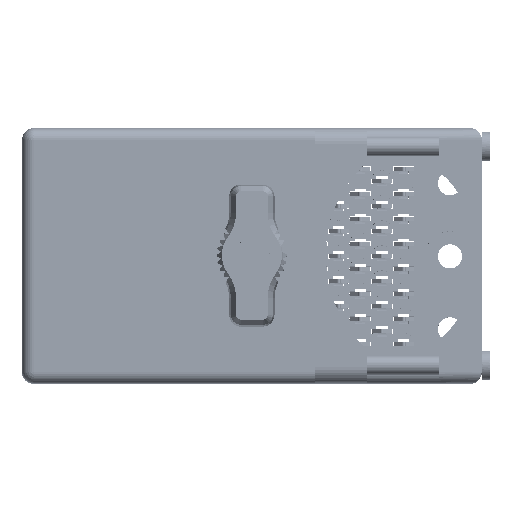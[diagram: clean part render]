
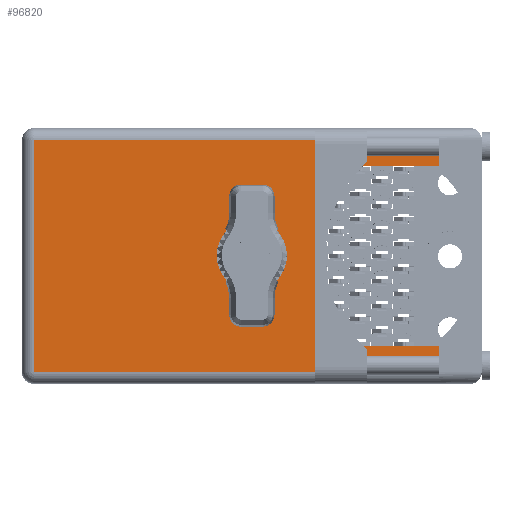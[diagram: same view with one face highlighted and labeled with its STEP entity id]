
A CAD part, top view. The second image highlights one B-rep face of the part: STEP entity #96820.
In plain terms, the highlighted face is planar.
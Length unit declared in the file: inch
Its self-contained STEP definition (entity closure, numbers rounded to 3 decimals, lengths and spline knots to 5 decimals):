
#288 = EDGE_CURVE ( 'NONE', #86348, #95004, #94879, .T. ) ;
#524 = CARTESIAN_POINT ( 'NONE',  ( 1.1215, 1.93, 0.54 ) ) ;
#705 = CARTESIAN_POINT ( 'NONE',  ( 1.1215, 1.93, 0.695 ) ) ;
#796 = ORIENTED_EDGE ( 'NONE', *, *, #88542, .T. ) ;
#2983 = VERTEX_POINT ( 'NONE', #27472 ) ;
#4107 = DIRECTION ( 'NONE',  ( -1., 0., 0. ) ) ;
#4232 = VECTOR ( 'NONE', #84432, 39.37008 ) ;
#4246 = CARTESIAN_POINT ( 'NONE',  ( 1.1215, 1.93, 0.54 ) ) ;
#7202 = DIRECTION ( 'NONE',  ( 1., 0., 0. ) ) ;
#8915 = CARTESIAN_POINT ( 'NONE',  ( 1.1215, 1.93, 0.695 ) ) ;
#9137 = DIRECTION ( 'NONE',  ( 0., 1., 0. ) ) ;
#14262 = VERTEX_POINT ( 'NONE', #8915 ) ;
#14741 = CARTESIAN_POINT ( 'NONE',  ( 0.4075, 1.93, 0.54 ) ) ;
#14955 = CARTESIAN_POINT ( 'NONE',  ( 0., 1.93, 0. ) ) ;
#16380 = ORIENTED_EDGE ( 'NONE', *, *, #67704, .T. ) ;
#16531 = ORIENTED_EDGE ( 'NONE', *, *, #102287, .T. ) ;
#17301 = DIRECTION ( 'NONE',  ( 0., 0., 1. ) ) ;
#17401 = EDGE_CURVE ( 'NONE', #102230, #2983, #83563, .T. ) ;
#18575 = CARTESIAN_POINT ( 'NONE',  ( 1.1215, 1.93, -0.765 ) ) ;
#19406 = VECTOR ( 'NONE', #26752, 39.37008 ) ;
#21004 = EDGE_LOOP ( 'NONE', ( #67143, #16531, #27596, #26174, #79886, #796, #93808, #16380 ) ) ;
#21429 = AXIS2_PLACEMENT_3D ( 'NONE', #82917, #9137, #17301 ) ;
#23336 = CARTESIAN_POINT ( 'NONE',  ( -1.3075, 1.93, -0.695 ) ) ;
#24018 = CARTESIAN_POINT ( 'NONE',  ( 0.4075, 1.93, -0.54 ) ) ;
#24276 = LINE ( 'NONE', #4246, #86844 ) ;
#25543 = ORIENTED_EDGE ( 'NONE', *, *, #105712, .F. ) ;
#25578 = DIRECTION ( 'NONE',  ( 0., 1., 0. ) ) ;
#26174 = ORIENTED_EDGE ( 'NONE', *, *, #61671, .T. ) ;
#26287 = DIRECTION ( 'NONE',  ( 0., 0., -1. ) ) ;
#26752 = DIRECTION ( 'NONE',  ( 1., 0., 0. ) ) ;
#27472 = CARTESIAN_POINT ( 'NONE',  ( 1.1215, 1.93, -0.54 ) ) ;
#27596 = ORIENTED_EDGE ( 'NONE', *, *, #50671, .F. ) ;
#31166 = DIRECTION ( 'NONE',  ( 0., 0., 1. ) ) ;
#34986 = DIRECTION ( 'NONE',  ( 0., 0., 1. ) ) ;
#36555 = PLANE ( 'NONE',  #62351 ) ;
#38083 = CARTESIAN_POINT ( 'NONE',  ( 0., 1.93, -0.17 ) ) ;
#39575 = LINE ( 'NONE', #705, #86782 ) ;
#39820 = EDGE_CURVE ( 'NONE', #99086, #43761, #62608, .T. ) ;
#40971 = CARTESIAN_POINT ( 'NONE',  ( 0., 1.93, 0.17 ) ) ;
#43761 = VERTEX_POINT ( 'NONE', #40971 ) ;
#48873 = VERTEX_POINT ( 'NONE', #524 ) ;
#49514 = LINE ( 'NONE', #69487, #53287 ) ;
#49958 = LINE ( 'NONE', #91996, #19406 ) ;
#50575 = ORIENTED_EDGE ( 'NONE', *, *, #39820, .F. ) ;
#50671 = EDGE_CURVE ( 'NONE', #48873, #14262, #61589, .T. ) ;
#52923 = DIRECTION ( 'NONE',  ( 0., 1., 0. ) ) ;
#53287 = VECTOR ( 'NONE', #85225, 39.37008 ) ;
#60062 = DIRECTION ( 'NONE',  ( 0., 0., 1. ) ) ;
#61589 = LINE ( 'NONE', #92238, #4232 ) ;
#61671 = EDGE_CURVE ( 'NONE', #48873, #86348, #24276, .T. ) ;
#62351 = AXIS2_PLACEMENT_3D ( 'NONE', #101777, #52923, #4107 ) ;
#62608 = CIRCLE ( 'NONE', #21429, 0.17 ) ;
#64220 = EDGE_LOOP ( 'NONE', ( #25543, #50575 ) ) ;
#65698 = CIRCLE ( 'NONE', #90373, 0.17 ) ;
#67143 = ORIENTED_EDGE ( 'NONE', *, *, #95298, .T. ) ;
#67704 = EDGE_CURVE ( 'NONE', #102230, #101703, #49514, .T. ) ;
#68015 = DIRECTION ( 'NONE',  ( -1., 0., 0. ) ) ;
#69487 = CARTESIAN_POINT ( 'NONE',  ( -1.3775, 1.93, -0.695 ) ) ;
#72274 = FACE_BOUND ( 'NONE', #64220, .T. ) ;
#73155 = VECTOR ( 'NONE', #26287, 39.37008 ) ;
#74495 = VECTOR ( 'NONE', #34986, 39.37008 ) ;
#74748 = FACE_OUTER_BOUND ( 'NONE', #21004, .T. ) ;
#79886 = ORIENTED_EDGE ( 'NONE', *, *, #288, .T. ) ;
#80039 = CARTESIAN_POINT ( 'NONE',  ( -1.3075, 1.93, -0.765 ) ) ;
#80666 = CARTESIAN_POINT ( 'NONE',  ( 1.1215, 1.93, -0.695 ) ) ;
#82917 = CARTESIAN_POINT ( 'NONE',  ( 0., 1.93, 0. ) ) ;
#83563 = LINE ( 'NONE', #18575, #74495 ) ;
#84432 = DIRECTION ( 'NONE',  ( 0., 0., 1. ) ) ;
#85225 = DIRECTION ( 'NONE',  ( -1., 0., 0. ) ) ;
#86348 = VERTEX_POINT ( 'NONE', #14741 ) ;
#86782 = VECTOR ( 'NONE', #7202, 39.37008 ) ;
#86844 = VECTOR ( 'NONE', #68015, 39.37008 ) ;
#88542 = EDGE_CURVE ( 'NONE', #95004, #2983, #49958, .T. ) ;
#90373 = AXIS2_PLACEMENT_3D ( 'NONE', #14955, #25578, #60062 ) ;
#90452 = VECTOR ( 'NONE', #31166, 39.37008 ) ;
#91663 = LINE ( 'NONE', #80039, #90452 ) ;
#91996 = CARTESIAN_POINT ( 'NONE',  ( 1.1215, 1.93, -0.54 ) ) ;
#92238 = CARTESIAN_POINT ( 'NONE',  ( 1.1215, 1.93, -0.765 ) ) ;
#92940 = CARTESIAN_POINT ( 'NONE',  ( 0.4075, 1.93, -0.54 ) ) ;
#93277 = CARTESIAN_POINT ( 'NONE',  ( -1.3075, 1.93, 0.695 ) ) ;
#93808 = ORIENTED_EDGE ( 'NONE', *, *, #17401, .F. ) ;
#94879 = LINE ( 'NONE', #92940, #73155 ) ;
#95004 = VERTEX_POINT ( 'NONE', #24018 ) ;
#95298 = EDGE_CURVE ( 'NONE', #101703, #101416, #91663, .T. ) ;
#96820 = ADVANCED_FACE ( 'NONE', ( #74748, #72274 ), #36555, .T. ) ;
#99086 = VERTEX_POINT ( 'NONE', #38083 ) ;
#101416 = VERTEX_POINT ( 'NONE', #93277 ) ;
#101703 = VERTEX_POINT ( 'NONE', #23336 ) ;
#101777 = CARTESIAN_POINT ( 'NONE',  ( -1.3775, 1.93, -0.765 ) ) ;
#102230 = VERTEX_POINT ( 'NONE', #80666 ) ;
#102287 = EDGE_CURVE ( 'NONE', #101416, #14262, #39575, .T. ) ;
#105712 = EDGE_CURVE ( 'NONE', #43761, #99086, #65698, .T. ) ;
